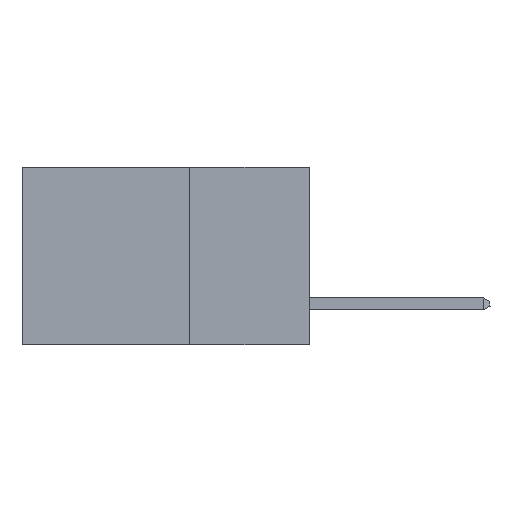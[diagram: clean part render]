
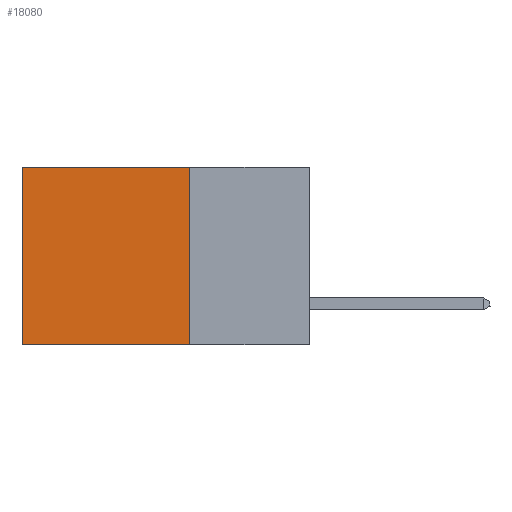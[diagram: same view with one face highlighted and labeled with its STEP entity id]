
A CAD part, left-side view. The second image highlights one B-rep face of the part: STEP entity #18080.
In plain terms, the highlighted planar face has unit normal (-1, 0, 0).
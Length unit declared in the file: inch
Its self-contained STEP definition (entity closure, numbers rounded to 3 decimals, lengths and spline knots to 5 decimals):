
#179 = LINE ( 'NONE', #4799, #23867 ) ;
#880 = CARTESIAN_POINT ( 'NONE',  ( 0.2875, 0.6, -0.37 ) ) ;
#1268 = CARTESIAN_POINT ( 'NONE',  ( 0.2875, 0.25, 0. ) ) ;
#1332 = VERTEX_POINT ( 'NONE', #13203 ) ;
#1884 = VERTEX_POINT ( 'NONE', #1268 ) ;
#1893 = DIRECTION ( 'NONE',  ( 0., 0., -1. ) ) ;
#2403 = ORIENTED_EDGE ( 'NONE', *, *, #20014, .T. ) ;
#3170 = ORIENTED_EDGE ( 'NONE', *, *, #26591, .F. ) ;
#3826 = DIRECTION ( 'NONE',  ( 1., 0., 0. ) ) ;
#4799 = CARTESIAN_POINT ( 'NONE',  ( 0.2875, 0.25, -0.37 ) ) ;
#5260 = EDGE_LOOP ( 'NONE', ( #2403, #3170, #26041, #12488 ) ) ;
#6097 = DIRECTION ( 'NONE',  ( 0., 0., -1. ) ) ;
#6738 = LINE ( 'NONE', #27026, #14608 ) ;
#7087 = DIRECTION ( 'NONE',  ( 0., 1., 0. ) ) ;
#8523 = PLANE ( 'NONE',  #22827 ) ;
#9324 = EDGE_CURVE ( 'NONE', #1884, #17376, #19280, .T. ) ;
#12488 = ORIENTED_EDGE ( 'NONE', *, *, #9324, .T. ) ;
#13203 = CARTESIAN_POINT ( 'NONE',  ( 0.2875, 0.25, -0.37 ) ) ;
#14608 = VECTOR ( 'NONE', #1893, 39.37008 ) ;
#15227 = CARTESIAN_POINT ( 'NONE',  ( 0.2875, 0.25, 0. ) ) ;
#15394 = FACE_OUTER_BOUND ( 'NONE', #5260, .T. ) ;
#17376 = VERTEX_POINT ( 'NONE', #28901 ) ;
#18080 = ADVANCED_FACE ( 'NONE', ( #15394 ), #8523, .F. ) ;
#18597 = EDGE_CURVE ( 'NONE', #1884, #1332, #6738, .T. ) ;
#19280 = LINE ( 'NONE', #26125, #27831 ) ;
#20014 = EDGE_CURVE ( 'NONE', #17376, #25024, #20860, .T. ) ;
#20860 = LINE ( 'NONE', #28008, #24391 ) ;
#22827 = AXIS2_PLACEMENT_3D ( 'NONE', #15227, #3826, #6097 ) ;
#23867 = VECTOR ( 'NONE', #7087, 39.37008 ) ;
#24391 = VECTOR ( 'NONE', #25867, 39.37008 ) ;
#25024 = VERTEX_POINT ( 'NONE', #880 ) ;
#25867 = DIRECTION ( 'NONE',  ( 0., 0., -1. ) ) ;
#26041 = ORIENTED_EDGE ( 'NONE', *, *, #18597, .F. ) ;
#26125 = CARTESIAN_POINT ( 'NONE',  ( 0.2875, 0.25, 0. ) ) ;
#26229 = DIRECTION ( 'NONE',  ( 0., 1., 0. ) ) ;
#26591 = EDGE_CURVE ( 'NONE', #1332, #25024, #179, .T. ) ;
#27026 = CARTESIAN_POINT ( 'NONE',  ( 0.2875, 0.25, 0. ) ) ;
#27831 = VECTOR ( 'NONE', #26229, 39.37008 ) ;
#28008 = CARTESIAN_POINT ( 'NONE',  ( 0.2875, 0.6, 0. ) ) ;
#28901 = CARTESIAN_POINT ( 'NONE',  ( 0.2875, 0.6, 0. ) ) ;
